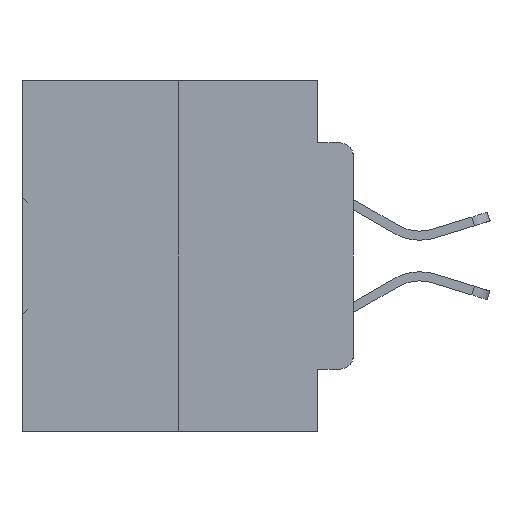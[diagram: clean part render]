
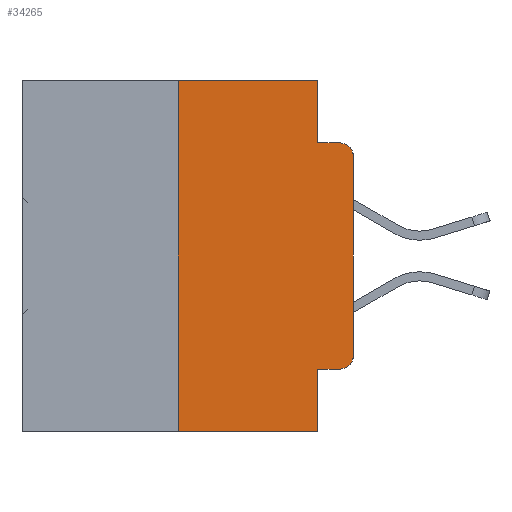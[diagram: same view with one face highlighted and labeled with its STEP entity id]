
A CAD part, left-side view. The second image highlights one B-rep face of the part: STEP entity #34265.
In plain terms, the highlighted planar face has unit normal (-1, 0, 0).
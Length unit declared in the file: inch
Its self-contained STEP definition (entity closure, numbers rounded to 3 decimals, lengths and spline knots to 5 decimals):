
#403 = EDGE_CURVE ( 'NONE', #21698, #8852, #16665, .T. ) ;
#516 = DIRECTION ( 'NONE',  ( -1., 0., 0. ) ) ;
#1147 = EDGE_LOOP ( 'NONE', ( #9418, #27203, #21688, #16979, #31109, #18377, #16782, #11556, #28508, #27322 ) ) ;
#1726 = VERTEX_POINT ( 'NONE', #6205 ) ;
#1885 = VERTEX_POINT ( 'NONE', #20206 ) ;
#2737 = DIRECTION ( 'NONE',  ( 0., 0., 1. ) ) ;
#3017 = VERTEX_POINT ( 'NONE', #27522 ) ;
#3763 = CARTESIAN_POINT ( 'NONE',  ( 0., 0., 0. ) ) ;
#4636 = DIRECTION ( 'NONE',  ( 0., -1., 0. ) ) ;
#4795 = DIRECTION ( 'NONE',  ( 0., -1., 0. ) ) ;
#5233 = EDGE_CURVE ( 'NONE', #3017, #27813, #20797, .T. ) ;
#6205 = CARTESIAN_POINT ( 'NONE',  ( 0., 0.051, -0.5 ) ) ;
#6574 = EDGE_CURVE ( 'NONE', #1885, #13764, #12036, .T. ) ;
#6777 = VECTOR ( 'NONE', #22612, 39.37008 ) ;
#6816 = AXIS2_PLACEMENT_3D ( 'NONE', #13656, #16331, #19071 ) ;
#6878 = EDGE_CURVE ( 'NONE', #21952, #30941, #25694, .T. ) ;
#7145 = VECTOR ( 'NONE', #4636, 39.37008 ) ;
#7417 = LINE ( 'NONE', #19875, #19005 ) ;
#8852 = VERTEX_POINT ( 'NONE', #25740 ) ;
#9418 = ORIENTED_EDGE ( 'NONE', *, *, #24379, .T. ) ;
#10352 = LINE ( 'NONE', #17161, #10734 ) ;
#10734 = VECTOR ( 'NONE', #4795, 39.37008 ) ;
#11004 = DIRECTION ( 'NONE',  ( 1., 0., 0. ) ) ;
#11161 = EDGE_CURVE ( 'NONE', #1885, #1726, #7417, .T. ) ;
#11556 = ORIENTED_EDGE ( 'NONE', *, *, #11161, .F. ) ;
#11885 = CARTESIAN_POINT ( 'NONE',  ( 0., 0.051, 0. ) ) ;
#12036 = LINE ( 'NONE', #19566, #29056 ) ;
#12791 = CARTESIAN_POINT ( 'NONE',  ( 0., 0., -0.3915 ) ) ;
#13656 = CARTESIAN_POINT ( 'NONE',  ( 0., 0.02, -0.1085 ) ) ;
#13764 = VERTEX_POINT ( 'NONE', #19780 ) ;
#13850 = CARTESIAN_POINT ( 'NONE',  ( 0., 0.25, 0. ) ) ;
#13946 = CARTESIAN_POINT ( 'NONE',  ( 0., 0.02, -0.0885 ) ) ;
#14298 = EDGE_CURVE ( 'NONE', #13764, #30373, #17255, .T. ) ;
#14850 = AXIS2_PLACEMENT_3D ( 'NONE', #26903, #11004, #21750 ) ;
#15396 = CARTESIAN_POINT ( 'NONE',  ( 0., 0.473, -0.5 ) ) ;
#16331 = DIRECTION ( 'NONE',  ( -1., 0., 0. ) ) ;
#16665 = LINE ( 'NONE', #13850, #17087 ) ;
#16782 = ORIENTED_EDGE ( 'NONE', *, *, #31554, .T. ) ;
#16979 = ORIENTED_EDGE ( 'NONE', *, *, #6878, .F. ) ;
#17087 = VECTOR ( 'NONE', #2737, 39.37008 ) ;
#17161 = CARTESIAN_POINT ( 'NONE',  ( 0., 0.473, 0. ) ) ;
#17255 = CIRCLE ( 'NONE', #33291, 0.02 ) ;
#17837 = VECTOR ( 'NONE', #32047, 39.37008 ) ;
#18377 = ORIENTED_EDGE ( 'NONE', *, *, #403, .F. ) ;
#18641 = VECTOR ( 'NONE', #23669, 39.37008 ) ;
#18723 = CARTESIAN_POINT ( 'NONE',  ( 0., 0.25, -0.5 ) ) ;
#18750 = EDGE_CURVE ( 'NONE', #30941, #27813, #19886, .T. ) ;
#19005 = VECTOR ( 'NONE', #22532, 39.37008 ) ;
#19049 = DIRECTION ( 'NONE',  ( 0., 0., -1. ) ) ;
#19071 = DIRECTION ( 'NONE',  ( 0., 0., -1. ) ) ;
#19566 = CARTESIAN_POINT ( 'NONE',  ( 0., 0.051, -0.4115 ) ) ;
#19780 = CARTESIAN_POINT ( 'NONE',  ( 0., 0.02, -0.4115 ) ) ;
#19875 = CARTESIAN_POINT ( 'NONE',  ( 0., 0.051, 0. ) ) ;
#19886 = LINE ( 'NONE', #21340, #17837 ) ;
#20206 = CARTESIAN_POINT ( 'NONE',  ( 0., 0.051, -0.4115 ) ) ;
#20396 = LINE ( 'NONE', #15396, #7145 ) ;
#20797 = CIRCLE ( 'NONE', #6816, 0.02 ) ;
#20882 = LINE ( 'NONE', #3763, #6777 ) ;
#21340 = CARTESIAN_POINT ( 'NONE',  ( 0., 0.051, -0.0885 ) ) ;
#21483 = CARTESIAN_POINT ( 'NONE',  ( 0., 0.02, -0.3915 ) ) ;
#21688 = ORIENTED_EDGE ( 'NONE', *, *, #18750, .F. ) ;
#21698 = VERTEX_POINT ( 'NONE', #18723 ) ;
#21750 = DIRECTION ( 'NONE',  ( 0., 0., -1. ) ) ;
#21952 = VERTEX_POINT ( 'NONE', #11885 ) ;
#22432 = FACE_OUTER_BOUND ( 'NONE', #1147, .T. ) ;
#22532 = DIRECTION ( 'NONE',  ( 0., 0., -1. ) ) ;
#22612 = DIRECTION ( 'NONE',  ( 0., 0., 1. ) ) ;
#23669 = DIRECTION ( 'NONE',  ( 0., 0., -1. ) ) ;
#24379 = EDGE_CURVE ( 'NONE', #30373, #3017, #20882, .T. ) ;
#25694 = LINE ( 'NONE', #26254, #18641 ) ;
#25740 = CARTESIAN_POINT ( 'NONE',  ( 0., 0.25, 0. ) ) ;
#25951 = CARTESIAN_POINT ( 'NONE',  ( 0., 0.051, -0.0885 ) ) ;
#26254 = CARTESIAN_POINT ( 'NONE',  ( 0., 0.051, 0. ) ) ;
#26903 = CARTESIAN_POINT ( 'NONE',  ( 0., 0.473, 0. ) ) ;
#26955 = EDGE_CURVE ( 'NONE', #8852, #21952, #10352, .T. ) ;
#27203 = ORIENTED_EDGE ( 'NONE', *, *, #5233, .T. ) ;
#27322 = ORIENTED_EDGE ( 'NONE', *, *, #14298, .T. ) ;
#27488 = DIRECTION ( 'NONE',  ( 0., -1., 0. ) ) ;
#27522 = CARTESIAN_POINT ( 'NONE',  ( 0., 0., -0.1085 ) ) ;
#27813 = VERTEX_POINT ( 'NONE', #13946 ) ;
#28508 = ORIENTED_EDGE ( 'NONE', *, *, #6574, .T. ) ;
#29056 = VECTOR ( 'NONE', #27488, 39.37008 ) ;
#30373 = VERTEX_POINT ( 'NONE', #12791 ) ;
#30941 = VERTEX_POINT ( 'NONE', #25951 ) ;
#31109 = ORIENTED_EDGE ( 'NONE', *, *, #26955, .F. ) ;
#31554 = EDGE_CURVE ( 'NONE', #21698, #1726, #20396, .T. ) ;
#32047 = DIRECTION ( 'NONE',  ( 0., -1., 0. ) ) ;
#32368 = PLANE ( 'NONE',  #14850 ) ;
#33291 = AXIS2_PLACEMENT_3D ( 'NONE', #21483, #516, #19049 ) ;
#34265 = ADVANCED_FACE ( 'NONE', ( #22432 ), #32368, .F. ) ;
